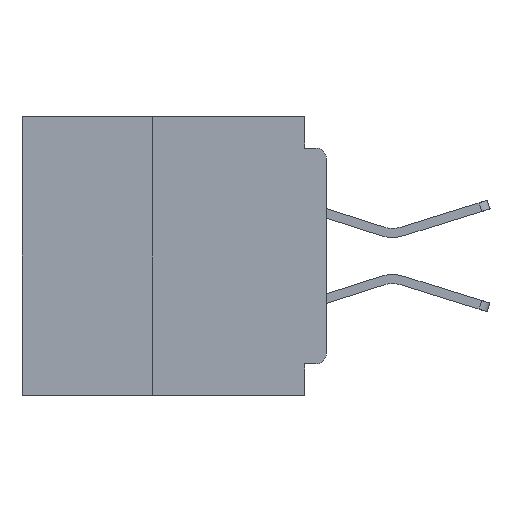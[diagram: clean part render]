
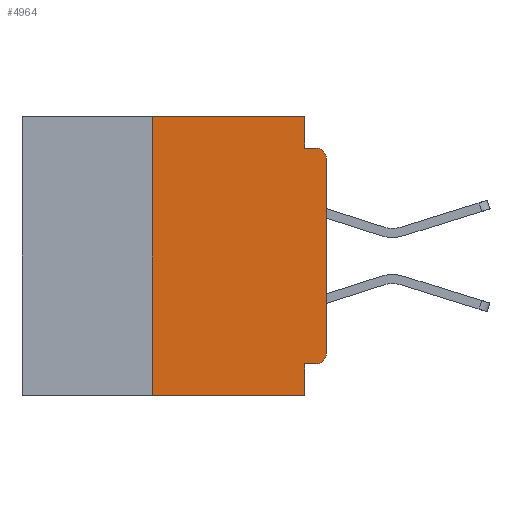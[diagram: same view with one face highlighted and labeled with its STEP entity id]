
A CAD part, left-side view. The second image highlights one B-rep face of the part: STEP entity #4964.
In plain terms, the highlighted planar face has unit normal (-1, 0, 0).
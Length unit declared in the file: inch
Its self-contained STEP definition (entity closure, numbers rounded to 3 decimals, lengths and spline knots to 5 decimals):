
#459 = AXIS2_PLACEMENT_3D ( 'NONE', #17320, #34459, #8829 ) ;
#860 = CARTESIAN_POINT ( 'NONE',  ( 0., 0., -0.355 ) ) ;
#1833 = ORIENTED_EDGE ( 'NONE', *, *, #34401, .T. ) ;
#2154 = CIRCLE ( 'NONE', #25200, 0.015 ) ;
#2526 = ORIENTED_EDGE ( 'NONE', *, *, #32900, .F. ) ;
#2727 = VECTOR ( 'NONE', #12626, 39.37008 ) ;
#2942 = EDGE_LOOP ( 'NONE', ( #29601, #48654, #37730, #49611, #2526, #50587, #39764, #16633, #53541, #1833 ) ) ;
#4458 = PLANE ( 'NONE',  #459 ) ;
#4964 = ADVANCED_FACE ( 'NONE', ( #25855 ), #4458, .F. ) ;
#5046 = CARTESIAN_POINT ( 'NONE',  ( 0., 0.031, 0. ) ) ;
#5242 = DIRECTION ( 'NONE',  ( 0., 1., 0. ) ) ;
#5739 = LINE ( 'NONE', #33268, #48417 ) ;
#5751 = CARTESIAN_POINT ( 'NONE',  ( 0., 0.015, -0.34 ) ) ;
#6823 = DIRECTION ( 'NONE',  ( 0., -1., 0. ) ) ;
#7466 = CARTESIAN_POINT ( 'NONE',  ( 0., 0., -0.06 ) ) ;
#7671 = VERTEX_POINT ( 'NONE', #5046 ) ;
#8600 = VECTOR ( 'NONE', #47999, 39.37008 ) ;
#8718 = LINE ( 'NONE', #32496, #31495 ) ;
#8818 = CARTESIAN_POINT ( 'NONE',  ( 0., 0.015, -0.045 ) ) ;
#8829 = DIRECTION ( 'NONE',  ( 0., 0., -1. ) ) ;
#9588 = CARTESIAN_POINT ( 'NONE',  ( 0., 0.25, -0.4 ) ) ;
#9716 = DIRECTION ( 'NONE',  ( 0., 0., 1. ) ) ;
#9846 = EDGE_CURVE ( 'NONE', #36241, #52569, #20057, .T. ) ;
#10141 = DIRECTION ( 'NONE',  ( 0., 0., -1. ) ) ;
#10867 = VERTEX_POINT ( 'NONE', #7466 ) ;
#11172 = DIRECTION ( 'NONE',  ( -1., 0., 0. ) ) ;
#12626 = DIRECTION ( 'NONE',  ( 0., 0., -1. ) ) ;
#14614 = VERTEX_POINT ( 'NONE', #19680 ) ;
#15756 = EDGE_CURVE ( 'NONE', #53386, #29969, #27921, .T. ) ;
#16444 = EDGE_CURVE ( 'NONE', #7671, #30551, #38542, .T. ) ;
#16629 = VECTOR ( 'NONE', #5242, 39.37008 ) ;
#16633 = ORIENTED_EDGE ( 'NONE', *, *, #28570, .F. ) ;
#17320 = CARTESIAN_POINT ( 'NONE',  ( 0., 0.437, 0. ) ) ;
#18755 = DIRECTION ( 'NONE',  ( 0., 0., -1. ) ) ;
#19680 = CARTESIAN_POINT ( 'NONE',  ( 0., 0.25, 0. ) ) ;
#20057 = LINE ( 'NONE', #39548, #8600 ) ;
#22884 = CARTESIAN_POINT ( 'NONE',  ( 0., 0.031, -0.4 ) ) ;
#24003 = CIRCLE ( 'NONE', #42076, 0.015 ) ;
#25200 = AXIS2_PLACEMENT_3D ( 'NONE', #5751, #35686, #10141 ) ;
#25611 = LINE ( 'NONE', #54964, #2727 ) ;
#25855 = FACE_OUTER_BOUND ( 'NONE', #2942, .T. ) ;
#25872 = VECTOR ( 'NONE', #18755, 39.37008 ) ;
#27227 = VERTEX_POINT ( 'NONE', #54728 ) ;
#27287 = CARTESIAN_POINT ( 'NONE',  ( 0., 0.031, 0. ) ) ;
#27921 = LINE ( 'NONE', #860, #16629 ) ;
#28570 = EDGE_CURVE ( 'NONE', #29969, #52569, #25611, .T. ) ;
#29601 = ORIENTED_EDGE ( 'NONE', *, *, #45944, .T. ) ;
#29969 = VERTEX_POINT ( 'NONE', #51480 ) ;
#30551 = VERTEX_POINT ( 'NONE', #38334 ) ;
#31495 = VECTOR ( 'NONE', #6823, 39.37008 ) ;
#32496 = CARTESIAN_POINT ( 'NONE',  ( 0., 0., -0.045 ) ) ;
#32900 = EDGE_CURVE ( 'NONE', #14614, #7671, #5739, .T. ) ;
#33268 = CARTESIAN_POINT ( 'NONE',  ( 0., 0.437, 0. ) ) ;
#34401 = EDGE_CURVE ( 'NONE', #53386, #27227, #2154, .T. ) ;
#34459 = DIRECTION ( 'NONE',  ( 1., 0., 0. ) ) ;
#35686 = DIRECTION ( 'NONE',  ( -1., 0., 0. ) ) ;
#36241 = VERTEX_POINT ( 'NONE', #9588 ) ;
#36703 = CARTESIAN_POINT ( 'NONE',  ( 0., 0.015, -0.06 ) ) ;
#36890 = EDGE_CURVE ( 'NONE', #36241, #14614, #49957, .T. ) ;
#37420 = VECTOR ( 'NONE', #9716, 39.37008 ) ;
#37641 = EDGE_CURVE ( 'NONE', #10867, #43347, #24003, .T. ) ;
#37730 = ORIENTED_EDGE ( 'NONE', *, *, #42454, .F. ) ;
#38221 = CARTESIAN_POINT ( 'NONE',  ( 0., 0., 0. ) ) ;
#38334 = CARTESIAN_POINT ( 'NONE',  ( 0., 0.031, -0.045 ) ) ;
#38405 = DIRECTION ( 'NONE',  ( 0., 0., 1. ) ) ;
#38542 = LINE ( 'NONE', #27287, #25872 ) ;
#39548 = CARTESIAN_POINT ( 'NONE',  ( 0., 0.437, -0.4 ) ) ;
#39728 = VECTOR ( 'NONE', #38405, 39.37008 ) ;
#39764 = ORIENTED_EDGE ( 'NONE', *, *, #9846, .T. ) ;
#41008 = DIRECTION ( 'NONE',  ( 0., 0., -1. ) ) ;
#42076 = AXIS2_PLACEMENT_3D ( 'NONE', #36703, #11172, #41008 ) ;
#42454 = EDGE_CURVE ( 'NONE', #30551, #43347, #8718, .T. ) ;
#43347 = VERTEX_POINT ( 'NONE', #8818 ) ;
#45944 = EDGE_CURVE ( 'NONE', #27227, #10867, #52240, .T. ) ;
#46031 = DIRECTION ( 'NONE',  ( 0., -1., 0. ) ) ;
#47999 = DIRECTION ( 'NONE',  ( 0., -1., 0. ) ) ;
#48417 = VECTOR ( 'NONE', #46031, 39.37008 ) ;
#48654 = ORIENTED_EDGE ( 'NONE', *, *, #37641, .T. ) ;
#49611 = ORIENTED_EDGE ( 'NONE', *, *, #16444, .F. ) ;
#49957 = LINE ( 'NONE', #52100, #37420 ) ;
#50587 = ORIENTED_EDGE ( 'NONE', *, *, #36890, .F. ) ;
#51480 = CARTESIAN_POINT ( 'NONE',  ( 0., 0.031, -0.355 ) ) ;
#52100 = CARTESIAN_POINT ( 'NONE',  ( 0., 0.25, -0.4 ) ) ;
#52240 = LINE ( 'NONE', #38221, #39728 ) ;
#52569 = VERTEX_POINT ( 'NONE', #22884 ) ;
#53386 = VERTEX_POINT ( 'NONE', #54318 ) ;
#53541 = ORIENTED_EDGE ( 'NONE', *, *, #15756, .F. ) ;
#54318 = CARTESIAN_POINT ( 'NONE',  ( 0., 0.015, -0.355 ) ) ;
#54728 = CARTESIAN_POINT ( 'NONE',  ( 0., 0., -0.34 ) ) ;
#54964 = CARTESIAN_POINT ( 'NONE',  ( 0., 0.031, -0.4 ) ) ;
